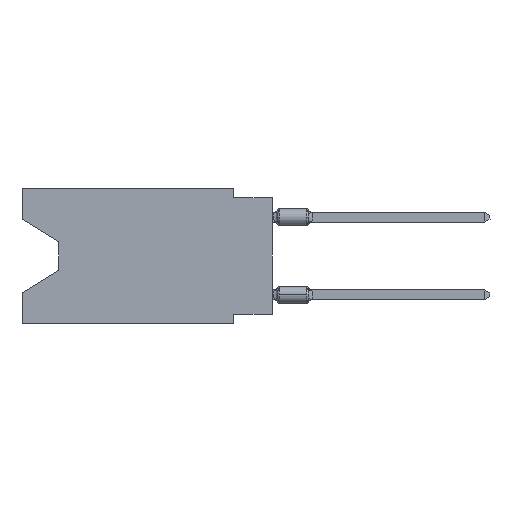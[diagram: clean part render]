
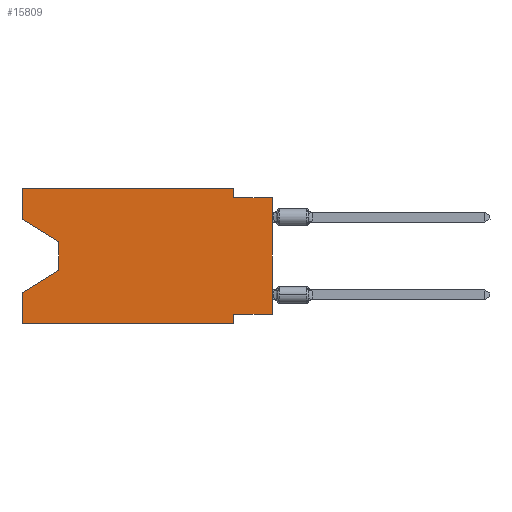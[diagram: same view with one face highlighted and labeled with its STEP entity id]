
A CAD part, left-side view. The second image highlights one B-rep face of the part: STEP entity #15809.
In plain terms, the highlighted planar face has unit normal (-1, 0, 0).
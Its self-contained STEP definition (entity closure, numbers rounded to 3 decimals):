
#436 = ORIENTED_EDGE ( 'NONE', *, *, #14012, .T. ) ;
#977 = DIRECTION ( 'NONE',  ( 0., 0., -1. ) ) ;
#1136 = DIRECTION ( 'NONE',  ( 0., 0., 1. ) ) ;
#1617 = EDGE_CURVE ( 'NONE', #4098, #16640, #18409, .T. ) ;
#1803 = AXIS2_PLACEMENT_3D ( 'NONE', #13424, #19994, #15247 ) ;
#1948 = EDGE_CURVE ( 'NONE', #6997, #7697, #2455, .T. ) ;
#2276 = CARTESIAN_POINT ( 'NONE',  ( 0., 2.54, -8.89 ) ) ;
#2455 = LINE ( 'NONE', #10407, #15270 ) ;
#2622 = CARTESIAN_POINT ( 'NONE',  ( 0., 0., 0. ) ) ;
#2769 = CARTESIAN_POINT ( 'NONE',  ( 0., 16.383, 0. ) ) ;
#3256 = CARTESIAN_POINT ( 'NONE',  ( 0., 16.383, 0. ) ) ;
#3335 = CARTESIAN_POINT ( 'NONE',  ( 0., 2.54, -0.635 ) ) ;
#3345 = FACE_OUTER_BOUND ( 'NONE', #4575, .T. ) ;
#3481 = DIRECTION ( 'NONE',  ( 0., -1., 0. ) ) ;
#3621 = CARTESIAN_POINT ( 'NONE',  ( 0., 16.383, 0. ) ) ;
#3771 = CARTESIAN_POINT ( 'NONE',  ( 0., 13.97, -3.505 ) ) ;
#3807 = EDGE_CURVE ( 'NONE', #13773, #19257, #6619, .T. ) ;
#4098 = VERTEX_POINT ( 'NONE', #21210 ) ;
#4134 = CARTESIAN_POINT ( 'NONE',  ( 0., 2.54, -8.89 ) ) ;
#4151 = CARTESIAN_POINT ( 'NONE',  ( 0., 0., -8.255 ) ) ;
#4494 = LINE ( 'NONE', #20717, #6170 ) ;
#4575 = EDGE_LOOP ( 'NONE', ( #9451, #436, #5881, #17477, #17570, #13367, #5838, #20741, #20688, #4579, #12655, #12377 ) ) ;
#4579 = ORIENTED_EDGE ( 'NONE', *, *, #3807, .F. ) ;
#4627 = VECTOR ( 'NONE', #20412, 1000. ) ;
#5036 = VECTOR ( 'NONE', #8448, 1000. ) ;
#5373 = CARTESIAN_POINT ( 'NONE',  ( 0., 0., -0.635 ) ) ;
#5838 = ORIENTED_EDGE ( 'NONE', *, *, #6293, .F. ) ;
#5881 = ORIENTED_EDGE ( 'NONE', *, *, #13337, .T. ) ;
#5889 = DIRECTION ( 'NONE',  ( 0., -1., 0. ) ) ;
#6170 = VECTOR ( 'NONE', #5889, 1000. ) ;
#6293 = EDGE_CURVE ( 'NONE', #7253, #19065, #18560, .T. ) ;
#6561 = CARTESIAN_POINT ( 'NONE',  ( 0., 0., -8.255 ) ) ;
#6619 = LINE ( 'NONE', #15984, #7437 ) ;
#6673 = LINE ( 'NONE', #8079, #19084 ) ;
#6997 = VERTEX_POINT ( 'NONE', #10463 ) ;
#7127 = EDGE_CURVE ( 'NONE', #7253, #7803, #19164, .T. ) ;
#7253 = VERTEX_POINT ( 'NONE', #6561 ) ;
#7381 = CARTESIAN_POINT ( 'NONE',  ( 0., 13.97, -5.385 ) ) ;
#7437 = VECTOR ( 'NONE', #7820, 1000. ) ;
#7618 = EDGE_CURVE ( 'NONE', #13897, #13773, #19896, .T. ) ;
#7697 = VERTEX_POINT ( 'NONE', #3771 ) ;
#7803 = VERTEX_POINT ( 'NONE', #5373 ) ;
#7820 = DIRECTION ( 'NONE',  ( 0., 0., -1. ) ) ;
#8042 = CARTESIAN_POINT ( 'NONE',  ( 0., 16.383, 0. ) ) ;
#8079 = CARTESIAN_POINT ( 'NONE',  ( 0., 13.97, -3.505 ) ) ;
#8448 = DIRECTION ( 'NONE',  ( 0., 0., 1. ) ) ;
#8489 = PLANE ( 'NONE',  #1803 ) ;
#8809 = VECTOR ( 'NONE', #3481, 1000. ) ;
#9385 = VERTEX_POINT ( 'NONE', #10192 ) ;
#9451 = ORIENTED_EDGE ( 'NONE', *, *, #1948, .T. ) ;
#9477 = DIRECTION ( 'NONE',  ( 0., 0., 1. ) ) ;
#10132 = VECTOR ( 'NONE', #9477, 1000. ) ;
#10192 = CARTESIAN_POINT ( 'NONE',  ( 0., 16.383, -6.852 ) ) ;
#10295 = CARTESIAN_POINT ( 'NONE',  ( 0., 13.97, -5.385 ) ) ;
#10407 = CARTESIAN_POINT ( 'NONE',  ( 0., 16.383, -2.038 ) ) ;
#10438 = LINE ( 'NONE', #2276, #12240 ) ;
#10463 = CARTESIAN_POINT ( 'NONE',  ( 0., 16.383, -2.038 ) ) ;
#10569 = EDGE_CURVE ( 'NONE', #6997, #13897, #13174, .T. ) ;
#11208 = CARTESIAN_POINT ( 'NONE',  ( 0., 2.54, 0. ) ) ;
#11737 = CARTESIAN_POINT ( 'NONE',  ( 0., 16.383, -8.89 ) ) ;
#11904 = DIRECTION ( 'NONE',  ( 0., -0.855, -0.519 ) ) ;
#12240 = VECTOR ( 'NONE', #977, 1000. ) ;
#12377 = ORIENTED_EDGE ( 'NONE', *, *, #10569, .F. ) ;
#12561 = VECTOR ( 'NONE', #1136, 1000. ) ;
#12655 = ORIENTED_EDGE ( 'NONE', *, *, #7618, .F. ) ;
#13174 = LINE ( 'NONE', #3621, #5036 ) ;
#13241 = DIRECTION ( 'NONE',  ( 0., 0., -1. ) ) ;
#13337 = EDGE_CURVE ( 'NONE', #19803, #9385, #15559, .T. ) ;
#13367 = ORIENTED_EDGE ( 'NONE', *, *, #18136, .F. ) ;
#13424 = CARTESIAN_POINT ( 'NONE',  ( 0., 16.383, 0. ) ) ;
#13773 = VERTEX_POINT ( 'NONE', #11208 ) ;
#13897 = VERTEX_POINT ( 'NONE', #3256 ) ;
#14012 = EDGE_CURVE ( 'NONE', #7697, #19803, #6673, .T. ) ;
#15247 = DIRECTION ( 'NONE',  ( 0., 0., -1. ) ) ;
#15270 = VECTOR ( 'NONE', #11904, 1000. ) ;
#15559 = LINE ( 'NONE', #7381, #4627 ) ;
#15809 = ADVANCED_FACE ( 'NONE', ( #3345 ), #8489, .F. ) ;
#15984 = CARTESIAN_POINT ( 'NONE',  ( 0., 2.54, 0. ) ) ;
#16640 = VERTEX_POINT ( 'NONE', #4134 ) ;
#16883 = CARTESIAN_POINT ( 'NONE',  ( 0., 2.54, -8.255 ) ) ;
#16939 = DIRECTION ( 'NONE',  ( 0., 1., 0. ) ) ;
#17477 = ORIENTED_EDGE ( 'NONE', *, *, #17628, .F. ) ;
#17570 = ORIENTED_EDGE ( 'NONE', *, *, #1617, .T. ) ;
#17628 = EDGE_CURVE ( 'NONE', #4098, #9385, #19089, .T. ) ;
#18136 = EDGE_CURVE ( 'NONE', #19065, #16640, #10438, .T. ) ;
#18161 = DIRECTION ( 'NONE',  ( 0., -1., 0. ) ) ;
#18409 = LINE ( 'NONE', #11737, #8809 ) ;
#18560 = LINE ( 'NONE', #4151, #20393 ) ;
#18718 = VECTOR ( 'NONE', #18161, 1000. ) ;
#19065 = VERTEX_POINT ( 'NONE', #16883 ) ;
#19084 = VECTOR ( 'NONE', #13241, 1000. ) ;
#19089 = LINE ( 'NONE', #2769, #12561 ) ;
#19164 = LINE ( 'NONE', #2622, #10132 ) ;
#19257 = VERTEX_POINT ( 'NONE', #3335 ) ;
#19803 = VERTEX_POINT ( 'NONE', #10295 ) ;
#19896 = LINE ( 'NONE', #8042, #18718 ) ;
#19994 = DIRECTION ( 'NONE',  ( 1., 0., 0. ) ) ;
#20393 = VECTOR ( 'NONE', #16939, 1000. ) ;
#20412 = DIRECTION ( 'NONE',  ( 0., 0.855, -0.519 ) ) ;
#20634 = EDGE_CURVE ( 'NONE', #19257, #7803, #4494, .T. ) ;
#20688 = ORIENTED_EDGE ( 'NONE', *, *, #20634, .F. ) ;
#20717 = CARTESIAN_POINT ( 'NONE',  ( 0., 0., -0.635 ) ) ;
#20741 = ORIENTED_EDGE ( 'NONE', *, *, #7127, .T. ) ;
#21210 = CARTESIAN_POINT ( 'NONE',  ( 0., 16.383, -8.89 ) ) ;
